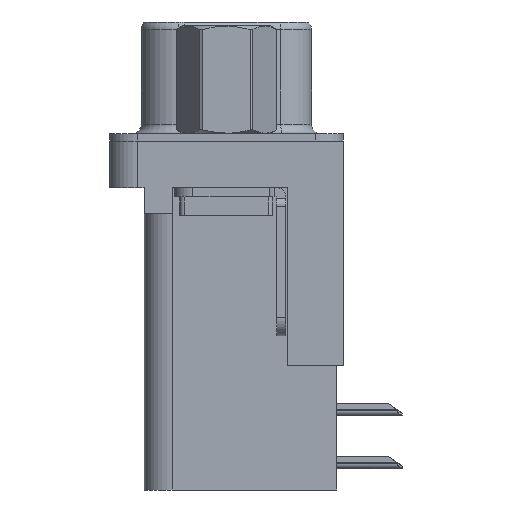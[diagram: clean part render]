
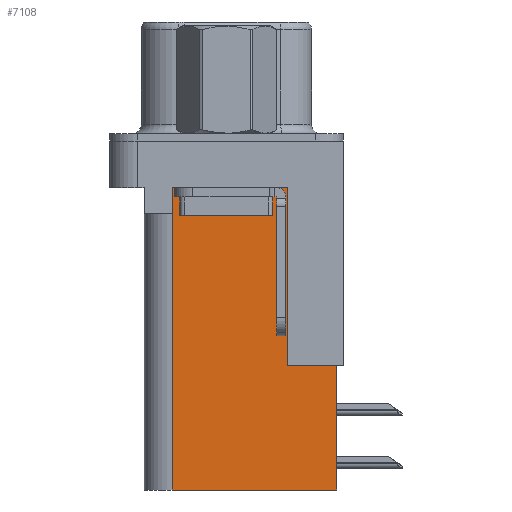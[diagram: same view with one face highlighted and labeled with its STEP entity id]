
A CAD part, left-side view. The second image highlights one B-rep face of the part: STEP entity #7108.
In plain terms, the highlighted planar face has unit normal (-1, 0, 0).
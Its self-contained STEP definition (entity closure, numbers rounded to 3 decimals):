
#45 = ORIENTED_EDGE ( 'NONE', *, *, #17423, .T. ) ;
#176 = VERTEX_POINT ( 'NONE', #11394 ) ;
#818 = EDGE_CURVE ( 'NONE', #17957, #4528, #11503, .T. ) ;
#1393 = AXIS2_PLACEMENT_3D ( 'NONE', #8490, #19250, #6463 ) ;
#1495 = CARTESIAN_POINT ( 'NONE',  ( 3.7, 2.895, -3.9 ) ) ;
#1636 = ORIENTED_EDGE ( 'NONE', *, *, #1877, .T. ) ;
#1873 = ORIENTED_EDGE ( 'NONE', *, *, #23880, .T. ) ;
#1877 = EDGE_CURVE ( 'NONE', #176, #24657, #12779, .T. ) ;
#1956 = DIRECTION ( 'NONE',  ( 0., 1., 0. ) ) ;
#2808 = ORIENTED_EDGE ( 'NONE', *, *, #4754, .F. ) ;
#3083 = LINE ( 'NONE', #14742, #8077 ) ;
#3135 = VECTOR ( 'NONE', #3620, 1000. ) ;
#3620 = DIRECTION ( 'NONE',  ( 0., 0., -1. ) ) ;
#3774 = VERTEX_POINT ( 'NONE', #15365 ) ;
#4099 = CARTESIAN_POINT ( 'NONE',  ( 3.7, 2.895, -3.9 ) ) ;
#4132 = ORIENTED_EDGE ( 'NONE', *, *, #818, .T. ) ;
#4528 = VERTEX_POINT ( 'NONE', #17411 ) ;
#4694 = CARTESIAN_POINT ( 'NONE',  ( 3.7, -3.295, -12.05 ) ) ;
#4754 = EDGE_CURVE ( 'NONE', #176, #3774, #14636, .T. ) ;
#5077 = CARTESIAN_POINT ( 'NONE',  ( 3.7, -3.295, -2.5 ) ) ;
#5480 = LINE ( 'NONE', #14789, #17507 ) ;
#6463 = DIRECTION ( 'NONE',  ( 0., 1., 0. ) ) ;
#7017 = VERTEX_POINT ( 'NONE', #4099 ) ;
#7108 = ADVANCED_FACE ( 'NONE', ( #18218 ), #14952, .F. ) ;
#7121 = VECTOR ( 'NONE', #10827, 1000. ) ;
#7244 = DIRECTION ( 'NONE',  ( 0., 0., 1. ) ) ;
#7502 = CARTESIAN_POINT ( 'NONE',  ( 3.7, 2.925, -3.9 ) ) ;
#7625 = VECTOR ( 'NONE', #9151, 1000. ) ;
#8077 = VECTOR ( 'NONE', #1956, 1000. ) ;
#8490 = CARTESIAN_POINT ( 'NONE',  ( 3.7, -3.295, -18.76 ) ) ;
#8901 = VERTEX_POINT ( 'NONE', #7502 ) ;
#9035 = EDGE_CURVE ( 'NONE', #3774, #9444, #3083, .T. ) ;
#9151 = DIRECTION ( 'NONE',  ( 0., 0., -1. ) ) ;
#9231 = LINE ( 'NONE', #15658, #25547 ) ;
#9444 = VERTEX_POINT ( 'NONE', #9595 ) ;
#9595 = CARTESIAN_POINT ( 'NONE',  ( 3.7, 2.925, -18.76 ) ) ;
#10172 = VECTOR ( 'NONE', #14438, 1000. ) ;
#10827 = DIRECTION ( 'NONE',  ( 0., 1., 0. ) ) ;
#10891 = VECTOR ( 'NONE', #16665, 1000. ) ;
#11394 = CARTESIAN_POINT ( 'NONE',  ( 3.7, -5.925, -12.05 ) ) ;
#11503 = LINE ( 'NONE', #23172, #10172 ) ;
#12659 = EDGE_LOOP ( 'NONE', ( #4132, #45, #23117, #23639, #15487, #2808, #1636, #1873 ) ) ;
#12779 = LINE ( 'NONE', #13281, #7121 ) ;
#13281 = CARTESIAN_POINT ( 'NONE',  ( 3.7, -6.295, -12.05 ) ) ;
#14438 = DIRECTION ( 'NONE',  ( 0., 1., 0. ) ) ;
#14636 = LINE ( 'NONE', #21957, #7625 ) ;
#14742 = CARTESIAN_POINT ( 'NONE',  ( 3.7, -3.295, -18.76 ) ) ;
#14789 = CARTESIAN_POINT ( 'NONE',  ( 3.7, 0., -3.9 ) ) ;
#14952 = PLANE ( 'NONE',  #1393 ) ;
#15365 = CARTESIAN_POINT ( 'NONE',  ( 3.7, -5.925, -18.76 ) ) ;
#15487 = ORIENTED_EDGE ( 'NONE', *, *, #9035, .F. ) ;
#15658 = CARTESIAN_POINT ( 'NONE',  ( 3.7, 2.925, -18.76 ) ) ;
#16665 = DIRECTION ( 'NONE',  ( 0., 0., 1. ) ) ;
#16935 = DIRECTION ( 'NONE',  ( 0., 1., 0. ) ) ;
#17411 = CARTESIAN_POINT ( 'NONE',  ( 3.7, 2.895, -2.5 ) ) ;
#17423 = EDGE_CURVE ( 'NONE', #4528, #7017, #24505, .T. ) ;
#17507 = VECTOR ( 'NONE', #16935, 1000. ) ;
#17957 = VERTEX_POINT ( 'NONE', #5077 ) ;
#18218 = FACE_OUTER_BOUND ( 'NONE', #12659, .T. ) ;
#19250 = DIRECTION ( 'NONE',  ( 1., 0., 0. ) ) ;
#21957 = CARTESIAN_POINT ( 'NONE',  ( 3.7, -5.925, -2. ) ) ;
#23108 = CARTESIAN_POINT ( 'NONE',  ( 3.7, -3.295, -18.76 ) ) ;
#23117 = ORIENTED_EDGE ( 'NONE', *, *, #25753, .T. ) ;
#23172 = CARTESIAN_POINT ( 'NONE',  ( 3.7, -3.295, -2.5 ) ) ;
#23639 = ORIENTED_EDGE ( 'NONE', *, *, #24252, .F. ) ;
#23880 = EDGE_CURVE ( 'NONE', #24657, #17957, #27186, .T. ) ;
#24252 = EDGE_CURVE ( 'NONE', #9444, #8901, #9231, .T. ) ;
#24505 = LINE ( 'NONE', #1495, #3135 ) ;
#24657 = VERTEX_POINT ( 'NONE', #4694 ) ;
#25547 = VECTOR ( 'NONE', #7244, 1000. ) ;
#25753 = EDGE_CURVE ( 'NONE', #7017, #8901, #5480, .T. ) ;
#27186 = LINE ( 'NONE', #23108, #10891 ) ;
